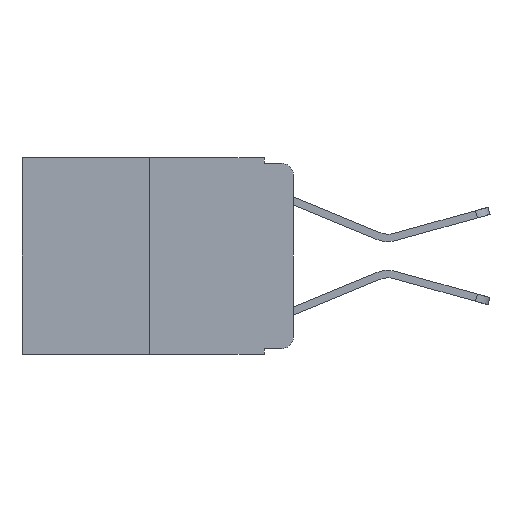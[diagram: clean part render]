
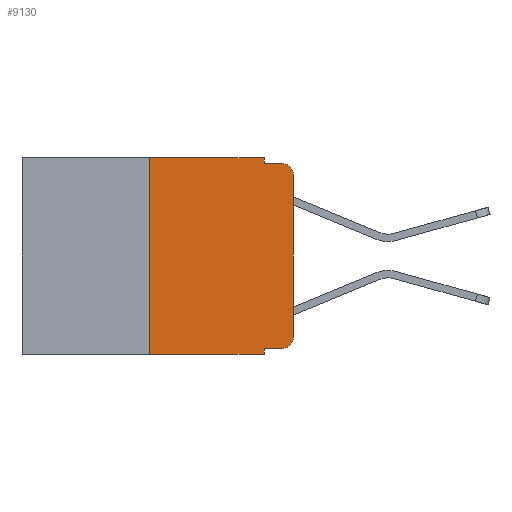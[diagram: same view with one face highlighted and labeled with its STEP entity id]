
A CAD part, left-side view. The second image highlights one B-rep face of the part: STEP entity #9130.
In plain terms, the highlighted planar face has unit normal (-1, 0, 0).
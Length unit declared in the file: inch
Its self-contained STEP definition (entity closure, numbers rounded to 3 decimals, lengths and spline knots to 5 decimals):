
#245 = EDGE_LOOP ( 'NONE', ( #6285, #6356, #6343, #6444, #6226, #9556, #9435, #9658, #6115, #9501 ) ) ;
#265 = DIRECTION ( 'NONE',  ( 0., 0., 1. ) ) ;
#267 = EDGE_CURVE ( 'NONE', #6461, #10572, #9158, .T. ) ;
#360 = DIRECTION ( 'NONE',  ( -1., 0., 0. ) ) ;
#386 = DIRECTION ( 'NONE',  ( 0., 0., -1. ) ) ;
#441 = CARTESIAN_POINT ( 'NONE',  ( 0., 0.051, -0.343 ) ) ;
#649 = EDGE_CURVE ( 'NONE', #7712, #8458, #8448, .T. ) ;
#703 = VERTEX_POINT ( 'NONE', #7054 ) ;
#913 = CARTESIAN_POINT ( 'NONE',  ( 0., 0.473, -0.343 ) ) ;
#1787 = LINE ( 'NONE', #913, #4140 ) ;
#1922 = VERTEX_POINT ( 'NONE', #4863 ) ;
#1956 = VERTEX_POINT ( 'NONE', #9784 ) ;
#2030 = EDGE_CURVE ( 'NONE', #1922, #6461, #2499, .T. ) ;
#2055 = PLANE ( 'NONE',  #9487 ) ;
#2099 = DIRECTION ( 'NONE',  ( 0., -1., 0. ) ) ;
#2215 = VECTOR ( 'NONE', #11454, 39.37008 ) ;
#2357 = EDGE_CURVE ( 'NONE', #1922, #9663, #9950, .T. ) ;
#2370 = DIRECTION ( 'NONE',  ( 0., -1., 0. ) ) ;
#2411 = CARTESIAN_POINT ( 'NONE',  ( 0., 0.051, 0. ) ) ;
#2499 = LINE ( 'NONE', #11514, #8990 ) ;
#2583 = VERTEX_POINT ( 'NONE', #6345 ) ;
#2778 = EDGE_CURVE ( 'NONE', #1956, #5589, #11083, .T. ) ;
#2790 = CARTESIAN_POINT ( 'NONE',  ( 0., 0.25, 0. ) ) ;
#2919 = CARTESIAN_POINT ( 'NONE',  ( 0., 0.02, -0.333 ) ) ;
#3057 = CARTESIAN_POINT ( 'NONE',  ( 0., 0.473, 0. ) ) ;
#3126 = VECTOR ( 'NONE', #9042, 39.37008 ) ;
#4053 = DIRECTION ( 'NONE',  ( 0., 0., -1. ) ) ;
#4140 = VECTOR ( 'NONE', #8296, 39.37008 ) ;
#4227 = CARTESIAN_POINT ( 'NONE',  ( 0., 0., -0.313 ) ) ;
#4288 = VECTOR ( 'NONE', #265, 39.37008 ) ;
#4391 = DIRECTION ( 'NONE',  ( -1., 0., 0. ) ) ;
#4633 = LINE ( 'NONE', #2411, #10344 ) ;
#4863 = CARTESIAN_POINT ( 'NONE',  ( 0., 0.051, -0.333 ) ) ;
#5131 = DIRECTION ( 'NONE',  ( 0., -1., 0. ) ) ;
#5393 = DIRECTION ( 'NONE',  ( 0., 0., -1. ) ) ;
#5589 = VERTEX_POINT ( 'NONE', #2790 ) ;
#6115 = ORIENTED_EDGE ( 'NONE', *, *, #2030, .T. ) ;
#6179 = CARTESIAN_POINT ( 'NONE',  ( 0., 0., 0. ) ) ;
#6226 = ORIENTED_EDGE ( 'NONE', *, *, #9149, .F. ) ;
#6285 = ORIENTED_EDGE ( 'NONE', *, *, #8305, .T. ) ;
#6343 = ORIENTED_EDGE ( 'NONE', *, *, #8322, .F. ) ;
#6345 = CARTESIAN_POINT ( 'NONE',  ( 0., 0.051, -0.01 ) ) ;
#6356 = ORIENTED_EDGE ( 'NONE', *, *, #649, .T. ) ;
#6392 = AXIS2_PLACEMENT_3D ( 'NONE', #10029, #360, #386 ) ;
#6444 = ORIENTED_EDGE ( 'NONE', *, *, #8369, .F. ) ;
#6461 = VERTEX_POINT ( 'NONE', #2919 ) ;
#6495 = EDGE_CURVE ( 'NONE', #1956, #9663, #1787, .T. ) ;
#6751 = CARTESIAN_POINT ( 'NONE',  ( 0., 0.25, 0. ) ) ;
#6998 = FACE_OUTER_BOUND ( 'NONE', #245, .T. ) ;
#7024 = CARTESIAN_POINT ( 'NONE',  ( 0., 0.051, -0.01 ) ) ;
#7054 = CARTESIAN_POINT ( 'NONE',  ( 0., 0.051, 0. ) ) ;
#7202 = LINE ( 'NONE', #7024, #10601 ) ;
#7455 = CARTESIAN_POINT ( 'NONE',  ( 0., 0., -0.03 ) ) ;
#7504 = LINE ( 'NONE', #7612, #11163 ) ;
#7581 = AXIS2_PLACEMENT_3D ( 'NONE', #7932, #4391, #9365 ) ;
#7612 = CARTESIAN_POINT ( 'NONE',  ( 0., 0.473, 0. ) ) ;
#7712 = VERTEX_POINT ( 'NONE', #7455 ) ;
#7932 = CARTESIAN_POINT ( 'NONE',  ( 0., 0.02, -0.313 ) ) ;
#8265 = CARTESIAN_POINT ( 'NONE',  ( 0., 0.051, 0. ) ) ;
#8296 = DIRECTION ( 'NONE',  ( 0., -1., 0. ) ) ;
#8305 = EDGE_CURVE ( 'NONE', #10572, #7712, #10854, .T. ) ;
#8322 = EDGE_CURVE ( 'NONE', #2583, #8458, #7202, .T. ) ;
#8369 = EDGE_CURVE ( 'NONE', #703, #2583, #4633, .T. ) ;
#8448 = CIRCLE ( 'NONE', #6392, 0.02 ) ;
#8458 = VERTEX_POINT ( 'NONE', #10216 ) ;
#8990 = VECTOR ( 'NONE', #5131, 39.37008 ) ;
#9042 = DIRECTION ( 'NONE',  ( 0., 0., -1. ) ) ;
#9130 = ADVANCED_FACE ( 'NONE', ( #6998 ), #2055, .F. ) ;
#9144 = DIRECTION ( 'NONE',  ( 1., 0., 0. ) ) ;
#9149 = EDGE_CURVE ( 'NONE', #5589, #703, #7504, .T. ) ;
#9158 = CIRCLE ( 'NONE', #7581, 0.02 ) ;
#9365 = DIRECTION ( 'NONE',  ( 0., 0., -1. ) ) ;
#9435 = ORIENTED_EDGE ( 'NONE', *, *, #6495, .T. ) ;
#9487 = AXIS2_PLACEMENT_3D ( 'NONE', #3057, #9144, #4053 ) ;
#9501 = ORIENTED_EDGE ( 'NONE', *, *, #267, .T. ) ;
#9556 = ORIENTED_EDGE ( 'NONE', *, *, #2778, .F. ) ;
#9658 = ORIENTED_EDGE ( 'NONE', *, *, #2357, .F. ) ;
#9663 = VERTEX_POINT ( 'NONE', #441 ) ;
#9784 = CARTESIAN_POINT ( 'NONE',  ( 0., 0.25, -0.343 ) ) ;
#9950 = LINE ( 'NONE', #8265, #3126 ) ;
#10029 = CARTESIAN_POINT ( 'NONE',  ( 0., 0.02, -0.03 ) ) ;
#10216 = CARTESIAN_POINT ( 'NONE',  ( 0., 0.02, -0.01 ) ) ;
#10344 = VECTOR ( 'NONE', #5393, 39.37008 ) ;
#10572 = VERTEX_POINT ( 'NONE', #4227 ) ;
#10601 = VECTOR ( 'NONE', #2370, 39.37008 ) ;
#10854 = LINE ( 'NONE', #6179, #4288 ) ;
#11083 = LINE ( 'NONE', #6751, #2215 ) ;
#11163 = VECTOR ( 'NONE', #2099, 39.37008 ) ;
#11454 = DIRECTION ( 'NONE',  ( 0., 0., 1. ) ) ;
#11514 = CARTESIAN_POINT ( 'NONE',  ( 0., 0.051, -0.333 ) ) ;
